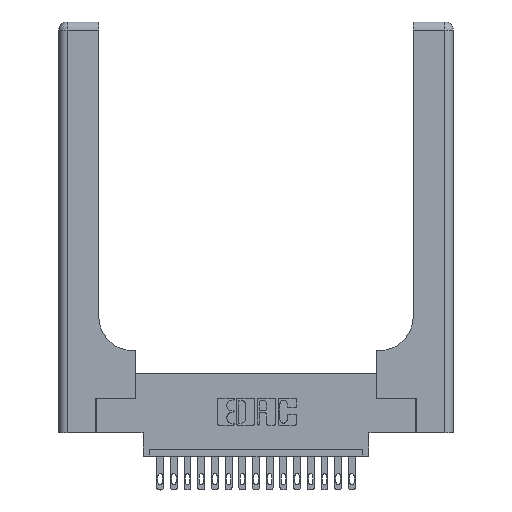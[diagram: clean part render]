
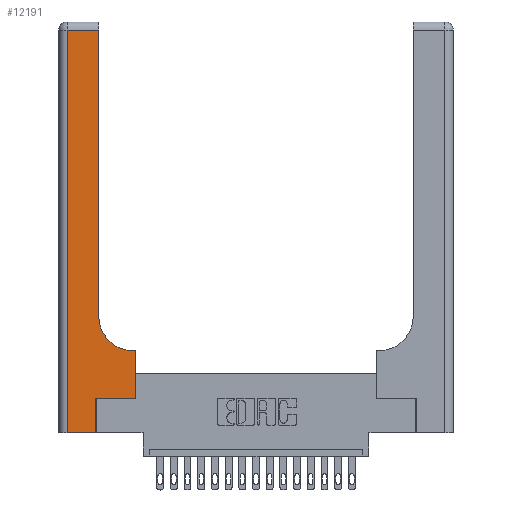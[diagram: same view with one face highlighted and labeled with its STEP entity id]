
A CAD part, top view. The second image highlights one B-rep face of the part: STEP entity #12191.
In plain terms, the highlighted planar face has unit normal (0, 0, 1).
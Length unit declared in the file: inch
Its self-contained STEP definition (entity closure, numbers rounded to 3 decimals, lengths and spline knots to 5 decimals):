
#964 = VERTEX_POINT ( 'NONE', #13313 ) ;
#1309 = EDGE_LOOP ( 'NONE', ( #16507, #16733, #17512, #12811, #16660, #11727, #15944, #9806, #13595 ) ) ;
#1341 = VERTEX_POINT ( 'NONE', #15190 ) ;
#1595 = VECTOR ( 'NONE', #9599, 39.37008 ) ;
#1881 = CARTESIAN_POINT ( 'NONE',  ( 0.06, 0., 0.37 ) ) ;
#2115 = EDGE_CURVE ( 'NONE', #17957, #13240, #18692, .T. ) ;
#2300 = CARTESIAN_POINT ( 'NONE',  ( 0.5585, 0.25, 0.37 ) ) ;
#2371 = EDGE_CURVE ( 'NONE', #1341, #13274, #15040, .T. ) ;
#3088 = LINE ( 'NONE', #18881, #1595 ) ;
#3442 = CARTESIAN_POINT ( 'NONE',  ( 0.5415, 0.6, 0.37 ) ) ;
#3477 = CARTESIAN_POINT ( 'NONE',  ( 0.2915, 0.85, 0.37 ) ) ;
#3825 = DIRECTION ( 'NONE',  ( 0., 0., -1. ) ) ;
#4130 = EDGE_CURVE ( 'NONE', #13274, #18076, #8433, .T. ) ;
#4491 = LINE ( 'NONE', #7733, #8877 ) ;
#4815 = CARTESIAN_POINT ( 'NONE',  ( 0.2915, 3., 0.37 ) ) ;
#4866 = CARTESIAN_POINT ( 'NONE',  ( 0.5585, 0.25, 0.37 ) ) ;
#5248 = VECTOR ( 'NONE', #19829, 39.37008 ) ;
#5396 = EDGE_CURVE ( 'NONE', #12332, #1341, #9597, .T. ) ;
#5437 = VECTOR ( 'NONE', #8062, 39.37008 ) ;
#6535 = CARTESIAN_POINT ( 'NONE',  ( 0.269, 0., 0.37 ) ) ;
#6562 = CARTESIAN_POINT ( 'NONE',  ( 0.06, 2.94, 0.37 ) ) ;
#6798 = VERTEX_POINT ( 'NONE', #1881 ) ;
#7622 = EDGE_CURVE ( 'NONE', #15385, #6798, #4491, .T. ) ;
#7733 = CARTESIAN_POINT ( 'NONE',  ( 0.06, 3., 0.37 ) ) ;
#8062 = DIRECTION ( 'NONE',  ( 0., 1., 0. ) ) ;
#8433 = CIRCLE ( 'NONE', #17133, 0.25 ) ;
#8877 = VECTOR ( 'NONE', #9297, 39.37008 ) ;
#9232 = VECTOR ( 'NONE', #9627, 39.37008 ) ;
#9297 = DIRECTION ( 'NONE',  ( 0., -1., 0. ) ) ;
#9597 = LINE ( 'NONE', #4866, #5437 ) ;
#9599 = DIRECTION ( 'NONE',  ( 1., 0., 0. ) ) ;
#9627 = DIRECTION ( 'NONE',  ( -1., 0., 0. ) ) ;
#9764 = CARTESIAN_POINT ( 'NONE',  ( 0.269, 0., 0.37 ) ) ;
#9806 = ORIENTED_EDGE ( 'NONE', *, *, #2371, .T. ) ;
#9890 = LINE ( 'NONE', #10602, #5248 ) ;
#9892 = PLANE ( 'NONE',  #12932 ) ;
#10602 = CARTESIAN_POINT ( 'NONE',  ( 0., 2.94, 0.37 ) ) ;
#10652 = FACE_OUTER_BOUND ( 'NONE', #1309, .T. ) ;
#11132 = EDGE_CURVE ( 'NONE', #13240, #12332, #16043, .T. ) ;
#11727 = ORIENTED_EDGE ( 'NONE', *, *, #11132, .T. ) ;
#12191 = ADVANCED_FACE ( 'NONE', ( #10652 ), #9892, .F. ) ;
#12332 = VERTEX_POINT ( 'NONE', #2300 ) ;
#12811 = ORIENTED_EDGE ( 'NONE', *, *, #18624, .T. ) ;
#12932 = AXIS2_PLACEMENT_3D ( 'NONE', #17897, #3825, #17706 ) ;
#13040 = EDGE_CURVE ( 'NONE', #964, #15385, #9890, .T. ) ;
#13240 = VERTEX_POINT ( 'NONE', #15536 ) ;
#13274 = VERTEX_POINT ( 'NONE', #3442 ) ;
#13285 = EDGE_CURVE ( 'NONE', #18076, #964, #15959, .T. ) ;
#13313 = CARTESIAN_POINT ( 'NONE',  ( 0.2915, 2.94, 0.37 ) ) ;
#13595 = ORIENTED_EDGE ( 'NONE', *, *, #4130, .T. ) ;
#14797 = CARTESIAN_POINT ( 'NONE',  ( 0.2915, 0.6, 0.37 ) ) ;
#14954 = CARTESIAN_POINT ( 'NONE',  ( 0.5415, 0.85, 0.37 ) ) ;
#15040 = LINE ( 'NONE', #14797, #9232 ) ;
#15190 = CARTESIAN_POINT ( 'NONE',  ( 0.5585, 0.6, 0.37 ) ) ;
#15385 = VERTEX_POINT ( 'NONE', #6562 ) ;
#15536 = CARTESIAN_POINT ( 'NONE',  ( 0.269, 0.25, 0.37 ) ) ;
#15641 = DIRECTION ( 'NONE',  ( 1., 0., 0. ) ) ;
#15944 = ORIENTED_EDGE ( 'NONE', *, *, #5396, .T. ) ;
#15959 = LINE ( 'NONE', #4815, #19078 ) ;
#16043 = LINE ( 'NONE', #20188, #17755 ) ;
#16507 = ORIENTED_EDGE ( 'NONE', *, *, #13285, .T. ) ;
#16660 = ORIENTED_EDGE ( 'NONE', *, *, #2115, .T. ) ;
#16733 = ORIENTED_EDGE ( 'NONE', *, *, #13040, .T. ) ;
#17133 = AXIS2_PLACEMENT_3D ( 'NONE', #14954, #17291, #15641 ) ;
#17291 = DIRECTION ( 'NONE',  ( 0., 0., -1. ) ) ;
#17512 = ORIENTED_EDGE ( 'NONE', *, *, #7622, .T. ) ;
#17706 = DIRECTION ( 'NONE',  ( -1., 0., 0. ) ) ;
#17755 = VECTOR ( 'NONE', #17885, 39.37008 ) ;
#17885 = DIRECTION ( 'NONE',  ( 1., 0., 0. ) ) ;
#17897 = CARTESIAN_POINT ( 'NONE',  ( 0., 3., 0.37 ) ) ;
#17957 = VERTEX_POINT ( 'NONE', #6535 ) ;
#18076 = VERTEX_POINT ( 'NONE', #3477 ) ;
#18451 = VECTOR ( 'NONE', #19376, 39.37008 ) ;
#18624 = EDGE_CURVE ( 'NONE', #6798, #17957, #3088, .T. ) ;
#18692 = LINE ( 'NONE', #9764, #18451 ) ;
#18881 = CARTESIAN_POINT ( 'NONE',  ( 0., 0., 0.37 ) ) ;
#18999 = DIRECTION ( 'NONE',  ( 0., 1., 0. ) ) ;
#19078 = VECTOR ( 'NONE', #18999, 39.37008 ) ;
#19376 = DIRECTION ( 'NONE',  ( 0., 1., 0. ) ) ;
#19829 = DIRECTION ( 'NONE',  ( -1., 0., 0. ) ) ;
#20188 = CARTESIAN_POINT ( 'NONE',  ( 0.269, 0.25, 0.37 ) ) ;
